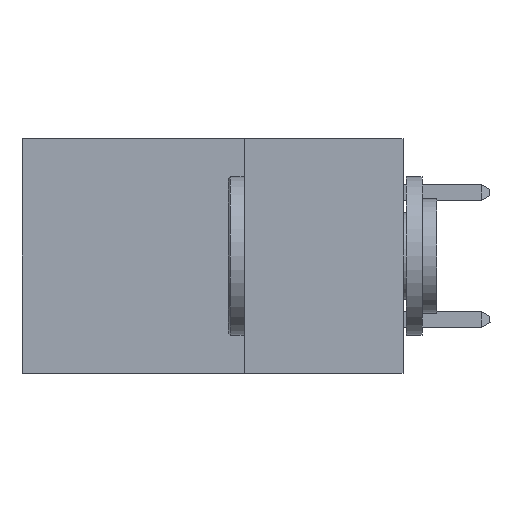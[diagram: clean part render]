
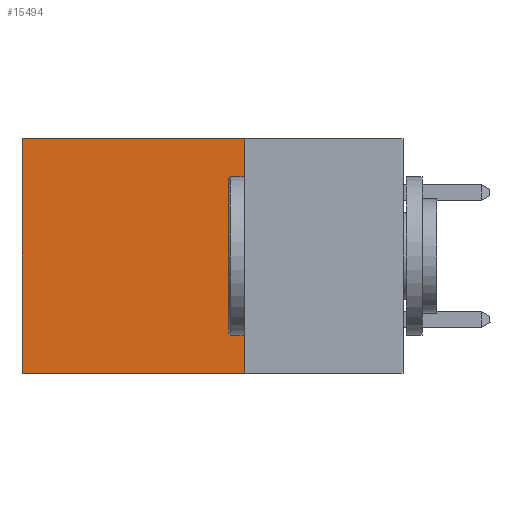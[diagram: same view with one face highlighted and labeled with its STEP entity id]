
A CAD part, left-side view. The second image highlights one B-rep face of the part: STEP entity #15494.
In plain terms, the highlighted planar face has unit normal (-1, 0, 0).
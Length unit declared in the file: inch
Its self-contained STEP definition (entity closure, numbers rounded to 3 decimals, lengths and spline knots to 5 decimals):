
#219 = CARTESIAN_POINT ( 'NONE',  ( 0.2875, 0.25, -0.37 ) ) ;
#1188 = ORIENTED_EDGE ( 'NONE', *, *, #17527, .F. ) ;
#2778 = CARTESIAN_POINT ( 'NONE',  ( 0.2875, 0.6, 0. ) ) ;
#4036 = EDGE_LOOP ( 'NONE', ( #20958, #1188, #19253, #6365 ) ) ;
#5593 = VECTOR ( 'NONE', #10796, 39.37008 ) ;
#5649 = CARTESIAN_POINT ( 'NONE',  ( 0.2875, 0.6, -0.37 ) ) ;
#6218 = DIRECTION ( 'NONE',  ( 0., 0., -1. ) ) ;
#6365 = ORIENTED_EDGE ( 'NONE', *, *, #13511, .T. ) ;
#7531 = VERTEX_POINT ( 'NONE', #219 ) ;
#8530 = DIRECTION ( 'NONE',  ( 0., 0., -1. ) ) ;
#8792 = LINE ( 'NONE', #9322, #5593 ) ;
#8795 = VERTEX_POINT ( 'NONE', #9516 ) ;
#9322 = CARTESIAN_POINT ( 'NONE',  ( 0.2875, 0.25, 0. ) ) ;
#9334 = LINE ( 'NONE', #2778, #18097 ) ;
#9516 = CARTESIAN_POINT ( 'NONE',  ( 0.2875, 0.25, 0. ) ) ;
#9825 = CARTESIAN_POINT ( 'NONE',  ( 0.2875, 0.25, 0. ) ) ;
#10796 = DIRECTION ( 'NONE',  ( 0., 1., 0. ) ) ;
#11744 = DIRECTION ( 'NONE',  ( 1., 0., 0. ) ) ;
#11758 = EDGE_CURVE ( 'NONE', #8795, #7531, #15741, .T. ) ;
#12371 = VERTEX_POINT ( 'NONE', #15015 ) ;
#12828 = VERTEX_POINT ( 'NONE', #5649 ) ;
#12961 = EDGE_CURVE ( 'NONE', #12371, #12828, #9334, .T. ) ;
#13511 = EDGE_CURVE ( 'NONE', #8795, #12371, #8792, .T. ) ;
#13561 = CARTESIAN_POINT ( 'NONE',  ( 0.2875, 0.25, 0. ) ) ;
#13857 = CARTESIAN_POINT ( 'NONE',  ( 0.2875, 0.25, -0.37 ) ) ;
#15015 = CARTESIAN_POINT ( 'NONE',  ( 0.2875, 0.6, 0. ) ) ;
#15194 = DIRECTION ( 'NONE',  ( 0., 0., -1. ) ) ;
#15494 = ADVANCED_FACE ( 'NONE', ( #20095 ), #18412, .F. ) ;
#15741 = LINE ( 'NONE', #13561, #21314 ) ;
#16959 = DIRECTION ( 'NONE',  ( 0., 1., 0. ) ) ;
#17113 = VECTOR ( 'NONE', #16959, 39.37008 ) ;
#17527 = EDGE_CURVE ( 'NONE', #7531, #12828, #18470, .T. ) ;
#18097 = VECTOR ( 'NONE', #6218, 39.37008 ) ;
#18412 = PLANE ( 'NONE',  #19560 ) ;
#18470 = LINE ( 'NONE', #13857, #17113 ) ;
#19253 = ORIENTED_EDGE ( 'NONE', *, *, #11758, .F. ) ;
#19560 = AXIS2_PLACEMENT_3D ( 'NONE', #9825, #11744, #15194 ) ;
#20095 = FACE_OUTER_BOUND ( 'NONE', #4036, .T. ) ;
#20958 = ORIENTED_EDGE ( 'NONE', *, *, #12961, .T. ) ;
#21314 = VECTOR ( 'NONE', #8530, 39.37008 ) ;
